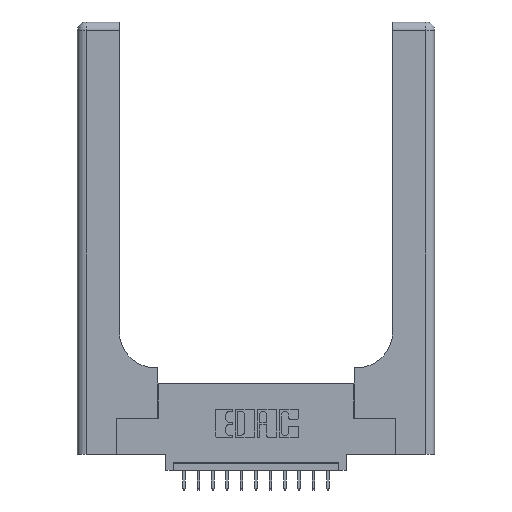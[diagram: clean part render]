
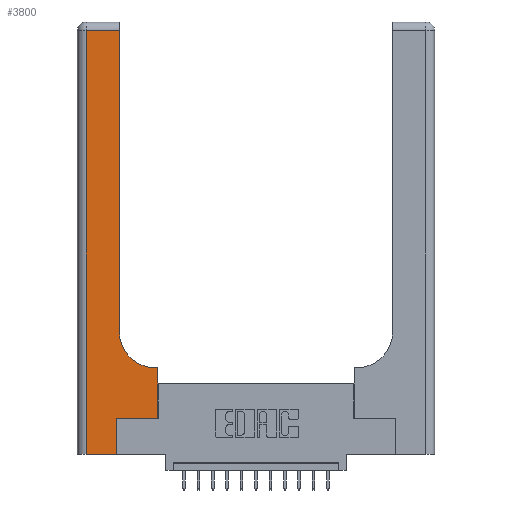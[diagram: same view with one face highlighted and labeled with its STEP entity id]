
A CAD part, top view. The second image highlights one B-rep face of the part: STEP entity #3800.
In plain terms, the highlighted planar face has unit normal (0, 0, 1).
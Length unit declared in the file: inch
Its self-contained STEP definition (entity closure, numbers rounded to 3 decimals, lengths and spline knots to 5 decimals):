
#2 = VERTEX_POINT ( 'NONE', #10797 ) ;
#104 = CARTESIAN_POINT ( 'NONE',  ( 0.2915, 2.94, 0.37 ) ) ;
#175 = VECTOR ( 'NONE', #2014, 39.37008 ) ;
#176 = VERTEX_POINT ( 'NONE', #9225 ) ;
#354 = CARTESIAN_POINT ( 'NONE',  ( 0., 2.94, 0.37 ) ) ;
#615 = CARTESIAN_POINT ( 'NONE',  ( 0.5585, 0.25, 0.37 ) ) ;
#1348 = AXIS2_PLACEMENT_3D ( 'NONE', #11984, #13246, #4987 ) ;
#1386 = EDGE_CURVE ( 'NONE', #14656, #2, #13240, .T. ) ;
#1528 = VERTEX_POINT ( 'NONE', #13847 ) ;
#1809 = LINE ( 'NONE', #14469, #6173 ) ;
#1895 = LINE ( 'NONE', #15647, #10458 ) ;
#2014 = DIRECTION ( 'NONE',  ( 0., 1., 0. ) ) ;
#2375 = CARTESIAN_POINT ( 'NONE',  ( 0.269, 0., 0.37 ) ) ;
#2396 = ORIENTED_EDGE ( 'NONE', *, *, #12344, .T. ) ;
#2439 = DIRECTION ( 'NONE',  ( 1., 0., 0. ) ) ;
#2548 = CARTESIAN_POINT ( 'NONE',  ( 0.2915, 0.6, 0.37 ) ) ;
#2769 = ORIENTED_EDGE ( 'NONE', *, *, #1386, .T. ) ;
#2973 = CARTESIAN_POINT ( 'NONE',  ( 0.2915, 0.85, 0.37 ) ) ;
#3058 = DIRECTION ( 'NONE',  ( -1., 0., 0. ) ) ;
#3468 = ORIENTED_EDGE ( 'NONE', *, *, #3798, .T. ) ;
#3798 = EDGE_CURVE ( 'NONE', #8752, #10884, #10704, .T. ) ;
#3800 = ADVANCED_FACE ( 'NONE', ( #12173 ), #5084, .F. ) ;
#3910 = VERTEX_POINT ( 'NONE', #104 ) ;
#3955 = VECTOR ( 'NONE', #11902, 39.37008 ) ;
#4398 = VECTOR ( 'NONE', #2439, 39.37008 ) ;
#4909 = ORIENTED_EDGE ( 'NONE', *, *, #12679, .T. ) ;
#4987 = DIRECTION ( 'NONE',  ( -1., 0., 0. ) ) ;
#5084 = PLANE ( 'NONE',  #1348 ) ;
#5903 = VECTOR ( 'NONE', #3058, 39.37008 ) ;
#6173 = VECTOR ( 'NONE', #7614, 39.37008 ) ;
#6956 = LINE ( 'NONE', #12205, #17135 ) ;
#7062 = CARTESIAN_POINT ( 'NONE',  ( 0.5415, 0.85, 0.37 ) ) ;
#7073 = VECTOR ( 'NONE', #17313, 39.37008 ) ;
#7614 = DIRECTION ( 'NONE',  ( 1., 0., 0. ) ) ;
#7971 = LINE ( 'NONE', #17512, #4398 ) ;
#8006 = ORIENTED_EDGE ( 'NONE', *, *, #12902, .T. ) ;
#8752 = VERTEX_POINT ( 'NONE', #13143 ) ;
#9103 = CARTESIAN_POINT ( 'NONE',  ( 0.5585, 0.25, 0.37 ) ) ;
#9225 = CARTESIAN_POINT ( 'NONE',  ( 0.06, 2.94, 0.37 ) ) ;
#9553 = DIRECTION ( 'NONE',  ( 0., 1., 0. ) ) ;
#9733 = ORIENTED_EDGE ( 'NONE', *, *, #17244, .T. ) ;
#9972 = EDGE_LOOP ( 'NONE', ( #8006, #16486, #15124, #9733, #2769, #2396, #12504, #3468, #4909 ) ) ;
#10451 = VERTEX_POINT ( 'NONE', #2973 ) ;
#10458 = VECTOR ( 'NONE', #12778, 39.37008 ) ;
#10704 = LINE ( 'NONE', #2548, #3955 ) ;
#10797 = CARTESIAN_POINT ( 'NONE',  ( 0.269, 0.25, 0.37 ) ) ;
#10884 = VERTEX_POINT ( 'NONE', #12774 ) ;
#11695 = CIRCLE ( 'NONE', #13995, 0.25 ) ;
#11902 = DIRECTION ( 'NONE',  ( -1., 0., 0. ) ) ;
#11984 = CARTESIAN_POINT ( 'NONE',  ( 0., 3., 0.37 ) ) ;
#12122 = EDGE_CURVE ( 'NONE', #176, #1528, #1895, .T. ) ;
#12173 = FACE_OUTER_BOUND ( 'NONE', #9972, .T. ) ;
#12205 = CARTESIAN_POINT ( 'NONE',  ( 0.2915, 3., 0.37 ) ) ;
#12344 = EDGE_CURVE ( 'NONE', #2, #12708, #7971, .T. ) ;
#12504 = ORIENTED_EDGE ( 'NONE', *, *, #12837, .T. ) ;
#12581 = DIRECTION ( 'NONE',  ( 1., 0., 0. ) ) ;
#12660 = CARTESIAN_POINT ( 'NONE',  ( 0.269, 0., 0.37 ) ) ;
#12679 = EDGE_CURVE ( 'NONE', #10884, #10451, #11695, .T. ) ;
#12708 = VERTEX_POINT ( 'NONE', #9103 ) ;
#12774 = CARTESIAN_POINT ( 'NONE',  ( 0.5415, 0.6, 0.37 ) ) ;
#12778 = DIRECTION ( 'NONE',  ( 0., -1., 0. ) ) ;
#12837 = EDGE_CURVE ( 'NONE', #12708, #8752, #13194, .T. ) ;
#12902 = EDGE_CURVE ( 'NONE', #10451, #3910, #6956, .T. ) ;
#13143 = CARTESIAN_POINT ( 'NONE',  ( 0.5585, 0.6, 0.37 ) ) ;
#13194 = LINE ( 'NONE', #615, #7073 ) ;
#13240 = LINE ( 'NONE', #2375, #175 ) ;
#13246 = DIRECTION ( 'NONE',  ( 0., 0., -1. ) ) ;
#13847 = CARTESIAN_POINT ( 'NONE',  ( 0.06, 0., 0.37 ) ) ;
#13995 = AXIS2_PLACEMENT_3D ( 'NONE', #7062, #14105, #12581 ) ;
#14105 = DIRECTION ( 'NONE',  ( 0., 0., -1. ) ) ;
#14469 = CARTESIAN_POINT ( 'NONE',  ( 0., 0., 0.37 ) ) ;
#14656 = VERTEX_POINT ( 'NONE', #12660 ) ;
#15124 = ORIENTED_EDGE ( 'NONE', *, *, #12122, .T. ) ;
#15444 = LINE ( 'NONE', #354, #5903 ) ;
#15647 = CARTESIAN_POINT ( 'NONE',  ( 0.06, 3., 0.37 ) ) ;
#16486 = ORIENTED_EDGE ( 'NONE', *, *, #17634, .T. ) ;
#17135 = VECTOR ( 'NONE', #9553, 39.37008 ) ;
#17244 = EDGE_CURVE ( 'NONE', #1528, #14656, #1809, .T. ) ;
#17313 = DIRECTION ( 'NONE',  ( 0., 1., 0. ) ) ;
#17512 = CARTESIAN_POINT ( 'NONE',  ( 0.269, 0.25, 0.37 ) ) ;
#17634 = EDGE_CURVE ( 'NONE', #3910, #176, #15444, .T. ) ;
